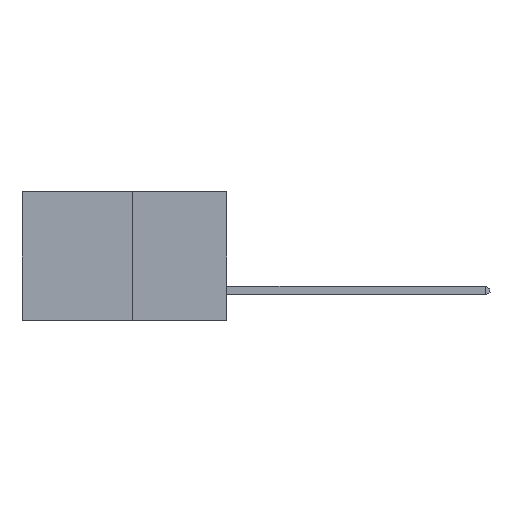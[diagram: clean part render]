
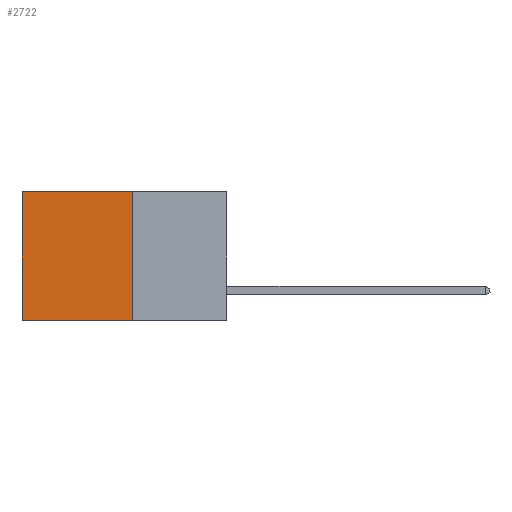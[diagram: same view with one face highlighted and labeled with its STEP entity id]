
A CAD part, left-side view. The second image highlights one B-rep face of the part: STEP entity #2722.
In plain terms, the highlighted planar face has unit normal (-1, 0, 0).
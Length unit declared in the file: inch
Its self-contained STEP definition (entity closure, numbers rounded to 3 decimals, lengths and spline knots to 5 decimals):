
#265 = FACE_OUTER_BOUND ( 'NONE', #6216, .T. ) ;
#301 = DIRECTION ( 'NONE',  ( 1., 0., 0. ) ) ;
#319 = DIRECTION ( 'NONE',  ( 0., 0., -1. ) ) ;
#545 = PLANE ( 'NONE',  #848 ) ;
#640 = LINE ( 'NONE', #4296, #2856 ) ;
#848 = AXIS2_PLACEMENT_3D ( 'NONE', #6469, #301, #319 ) ;
#1276 = CARTESIAN_POINT ( 'NONE',  ( 0.277, 0.59, 0. ) ) ;
#1532 = DIRECTION ( 'NONE',  ( 0., 0., -1. ) ) ;
#1683 = ORIENTED_EDGE ( 'NONE', *, *, #8865, .T. ) ;
#1870 = DIRECTION ( 'NONE',  ( 0., 0., -1. ) ) ;
#2087 = CARTESIAN_POINT ( 'NONE',  ( 0.277, 0.27, -0.37 ) ) ;
#2325 = CARTESIAN_POINT ( 'NONE',  ( 0.277, 0.27, -0.37 ) ) ;
#2545 = VERTEX_POINT ( 'NONE', #7644 ) ;
#2722 = ADVANCED_FACE ( 'NONE', ( #265 ), #545, .F. ) ;
#2780 = VERTEX_POINT ( 'NONE', #1276 ) ;
#2856 = VECTOR ( 'NONE', #1870, 39.37008 ) ;
#3342 = ORIENTED_EDGE ( 'NONE', *, *, #4919, .F. ) ;
#3672 = VECTOR ( 'NONE', #9856, 39.37008 ) ;
#3747 = CARTESIAN_POINT ( 'NONE',  ( 0.277, 0.59, -0.37 ) ) ;
#3850 = EDGE_CURVE ( 'NONE', #2780, #8032, #640, .T. ) ;
#3932 = LINE ( 'NONE', #9519, #3672 ) ;
#3982 = VERTEX_POINT ( 'NONE', #6054 ) ;
#4296 = CARTESIAN_POINT ( 'NONE',  ( 0.277, 0.59, -0.37 ) ) ;
#4919 = EDGE_CURVE ( 'NONE', #3982, #2545, #9465, .T. ) ;
#5013 = ORIENTED_EDGE ( 'NONE', *, *, #3850, .T. ) ;
#5457 = LINE ( 'NONE', #2087, #9403 ) ;
#5521 = VECTOR ( 'NONE', #1532, 39.37008 ) ;
#6054 = CARTESIAN_POINT ( 'NONE',  ( 0.277, 0.27, 0. ) ) ;
#6157 = DIRECTION ( 'NONE',  ( 0., 1., 0. ) ) ;
#6216 = EDGE_LOOP ( 'NONE', ( #5013, #7130, #3342, #1683 ) ) ;
#6469 = CARTESIAN_POINT ( 'NONE',  ( 0.277, 0.27, -0.37 ) ) ;
#7130 = ORIENTED_EDGE ( 'NONE', *, *, #9539, .F. ) ;
#7644 = CARTESIAN_POINT ( 'NONE',  ( 0.277, 0.27, -0.37 ) ) ;
#8032 = VERTEX_POINT ( 'NONE', #3747 ) ;
#8865 = EDGE_CURVE ( 'NONE', #3982, #2780, #3932, .T. ) ;
#9403 = VECTOR ( 'NONE', #6157, 39.37008 ) ;
#9465 = LINE ( 'NONE', #2325, #5521 ) ;
#9519 = CARTESIAN_POINT ( 'NONE',  ( 0.277, 0.27, 0. ) ) ;
#9539 = EDGE_CURVE ( 'NONE', #2545, #8032, #5457, .T. ) ;
#9856 = DIRECTION ( 'NONE',  ( 0., 1., 0. ) ) ;
